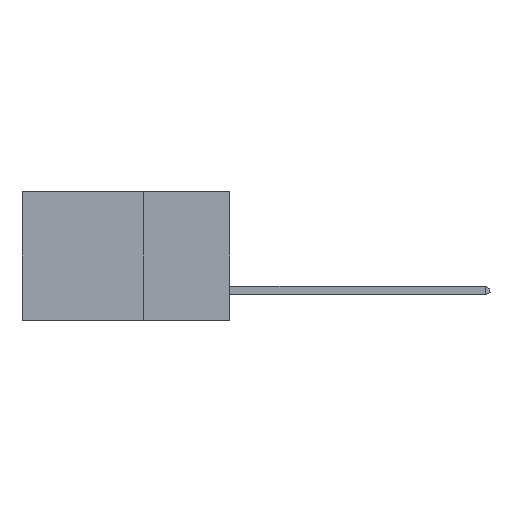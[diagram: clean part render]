
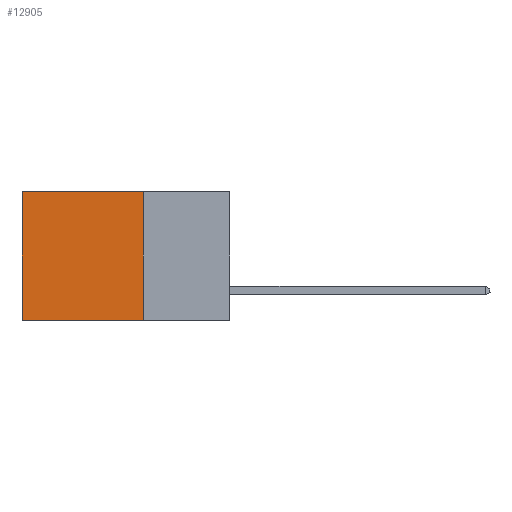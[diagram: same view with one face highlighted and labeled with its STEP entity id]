
A CAD part, left-side view. The second image highlights one B-rep face of the part: STEP entity #12905.
In plain terms, the highlighted planar face has unit normal (-1, 0, 0).
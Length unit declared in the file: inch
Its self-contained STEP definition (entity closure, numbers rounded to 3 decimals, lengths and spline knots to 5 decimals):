
#450 = EDGE_CURVE ( 'NONE', #13830, #13470, #10844, .T. ) ;
#750 = ORIENTED_EDGE ( 'NONE', *, *, #450, .T. ) ;
#914 = CARTESIAN_POINT ( 'NONE',  ( 0.298, 0.25, 0. ) ) ;
#1092 = CARTESIAN_POINT ( 'NONE',  ( 0.298, 0.25, 0. ) ) ;
#1096 = ORIENTED_EDGE ( 'NONE', *, *, #9427, .F. ) ;
#1202 = DIRECTION ( 'NONE',  ( 1., 0., 0. ) ) ;
#2640 = ORIENTED_EDGE ( 'NONE', *, *, #7030, .F. ) ;
#2962 = CARTESIAN_POINT ( 'NONE',  ( 0.298, 0.25, 0. ) ) ;
#3343 = DIRECTION ( 'NONE',  ( 0., 0., -1. ) ) ;
#4261 = CARTESIAN_POINT ( 'NONE',  ( 0.298, 0.25, -0.37 ) ) ;
#4305 = DIRECTION ( 'NONE',  ( 0., 1., 0. ) ) ;
#5575 = LINE ( 'NONE', #16870, #16548 ) ;
#5747 = VECTOR ( 'NONE', #3343, 39.37008 ) ;
#7030 = EDGE_CURVE ( 'NONE', #10195, #13470, #5575, .T. ) ;
#7910 = DIRECTION ( 'NONE',  ( 0., 0., -1. ) ) ;
#8489 = EDGE_CURVE ( 'NONE', #14061, #13830, #16958, .T. ) ;
#8540 = CARTESIAN_POINT ( 'NONE',  ( 0.298, 0.6, 0. ) ) ;
#8695 = DIRECTION ( 'NONE',  ( 0., 1., 0. ) ) ;
#9339 = CARTESIAN_POINT ( 'NONE',  ( 0.298, 0.25, 0. ) ) ;
#9427 = EDGE_CURVE ( 'NONE', #14061, #10195, #10993, .T. ) ;
#9822 = DIRECTION ( 'NONE',  ( 0., 0., -1. ) ) ;
#10043 = EDGE_LOOP ( 'NONE', ( #750, #2640, #1096, #17448 ) ) ;
#10046 = AXIS2_PLACEMENT_3D ( 'NONE', #9339, #1202, #7910 ) ;
#10195 = VERTEX_POINT ( 'NONE', #4261 ) ;
#10416 = VECTOR ( 'NONE', #4305, 39.37008 ) ;
#10662 = VECTOR ( 'NONE', #9822, 39.37008 ) ;
#10844 = LINE ( 'NONE', #16534, #10662 ) ;
#10993 = LINE ( 'NONE', #1092, #5747 ) ;
#11067 = FACE_OUTER_BOUND ( 'NONE', #10043, .T. ) ;
#11835 = PLANE ( 'NONE',  #10046 ) ;
#12905 = ADVANCED_FACE ( 'NONE', ( #11067 ), #11835, .F. ) ;
#12980 = CARTESIAN_POINT ( 'NONE',  ( 0.298, 0.6, -0.37 ) ) ;
#13470 = VERTEX_POINT ( 'NONE', #12980 ) ;
#13830 = VERTEX_POINT ( 'NONE', #8540 ) ;
#14061 = VERTEX_POINT ( 'NONE', #914 ) ;
#16534 = CARTESIAN_POINT ( 'NONE',  ( 0.298, 0.6, 0. ) ) ;
#16548 = VECTOR ( 'NONE', #8695, 39.37008 ) ;
#16870 = CARTESIAN_POINT ( 'NONE',  ( 0.298, 0.25, -0.37 ) ) ;
#16958 = LINE ( 'NONE', #2962, #10416 ) ;
#17448 = ORIENTED_EDGE ( 'NONE', *, *, #8489, .T. ) ;
